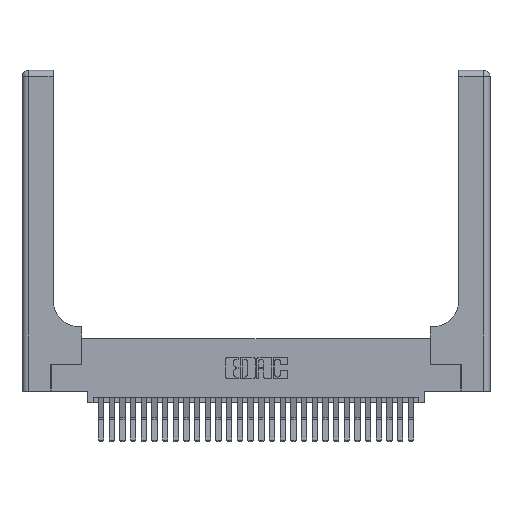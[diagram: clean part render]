
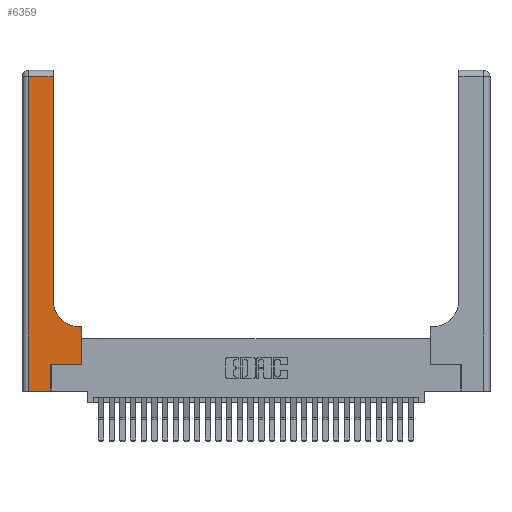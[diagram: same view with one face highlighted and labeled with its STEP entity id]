
A CAD part, top view. The second image highlights one B-rep face of the part: STEP entity #6359.
In plain terms, the highlighted planar face has unit normal (0, 0, 1).
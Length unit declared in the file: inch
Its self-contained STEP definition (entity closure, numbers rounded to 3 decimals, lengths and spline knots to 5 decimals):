
#84 = LINE ( 'NONE', #16524, #6353 ) ;
#564 = PLANE ( 'NONE',  #16732 ) ;
#703 = DIRECTION ( 'NONE',  ( 0., 1., 0. ) ) ;
#1130 = FACE_OUTER_BOUND ( 'NONE', #27902, .T. ) ;
#1442 = EDGE_CURVE ( 'NONE', #24325, #23639, #12715, .T. ) ;
#1774 = VERTEX_POINT ( 'NONE', #27814 ) ;
#1935 = DIRECTION ( 'NONE',  ( 1., 0., 0. ) ) ;
#2265 = DIRECTION ( 'NONE',  ( 1., 0., 0. ) ) ;
#2338 = CARTESIAN_POINT ( 'NONE',  ( 0., 2.94, 0.37 ) ) ;
#2570 = DIRECTION ( 'NONE',  ( -1., 0., 0. ) ) ;
#2942 = DIRECTION ( 'NONE',  ( 1., 0., 0. ) ) ;
#3468 = EDGE_CURVE ( 'NONE', #24528, #9712, #16293, .T. ) ;
#4187 = DIRECTION ( 'NONE',  ( 0., 0., -1. ) ) ;
#5060 = LINE ( 'NONE', #18318, #6574 ) ;
#5569 = EDGE_CURVE ( 'NONE', #18376, #21443, #25227, .T. ) ;
#5660 = ORIENTED_EDGE ( 'NONE', *, *, #5751, .T. ) ;
#5750 = CARTESIAN_POINT ( 'NONE',  ( 0.06, 2.94, 0.37 ) ) ;
#5751 = EDGE_CURVE ( 'NONE', #23639, #13401, #20760, .T. ) ;
#6353 = VECTOR ( 'NONE', #11831, 39.37008 ) ;
#6359 = ADVANCED_FACE ( 'NONE', ( #1130 ), #564, .F. ) ;
#6574 = VECTOR ( 'NONE', #25292, 39.37008 ) ;
#6883 = ORIENTED_EDGE ( 'NONE', *, *, #17012, .T. ) ;
#7183 = DIRECTION ( 'NONE',  ( -1., 0., 0. ) ) ;
#8137 = VECTOR ( 'NONE', #23333, 39.37008 ) ;
#9130 = ORIENTED_EDGE ( 'NONE', *, *, #1442, .T. ) ;
#9712 = VERTEX_POINT ( 'NONE', #17185 ) ;
#9992 = ORIENTED_EDGE ( 'NONE', *, *, #3468, .T. ) ;
#10165 = CARTESIAN_POINT ( 'NONE',  ( 0.269, 0., 0.37 ) ) ;
#10374 = VECTOR ( 'NONE', #2942, 39.37008 ) ;
#11231 = VECTOR ( 'NONE', #7183, 39.37008 ) ;
#11486 = EDGE_CURVE ( 'NONE', #21443, #1774, #5060, .T. ) ;
#11831 = DIRECTION ( 'NONE',  ( 0., 1., 0. ) ) ;
#11930 = CARTESIAN_POINT ( 'NONE',  ( 0.269, 0., 0.37 ) ) ;
#12715 = LINE ( 'NONE', #2338, #11231 ) ;
#13367 = CARTESIAN_POINT ( 'NONE',  ( 0.269, 0.25, 0.37 ) ) ;
#13401 = VERTEX_POINT ( 'NONE', #15048 ) ;
#13460 = CARTESIAN_POINT ( 'NONE',  ( 0., 3., 0.37 ) ) ;
#13659 = EDGE_CURVE ( 'NONE', #13401, #16905, #27153, .T. ) ;
#13711 = AXIS2_PLACEMENT_3D ( 'NONE', #16395, #21359, #2265 ) ;
#13730 = ORIENTED_EDGE ( 'NONE', *, *, #25328, .T. ) ;
#13891 = CARTESIAN_POINT ( 'NONE',  ( 0.06, 3., 0.37 ) ) ;
#14694 = CARTESIAN_POINT ( 'NONE',  ( 0.269, 0.25, 0.37 ) ) ;
#14718 = ORIENTED_EDGE ( 'NONE', *, *, #13659, .T. ) ;
#15048 = CARTESIAN_POINT ( 'NONE',  ( 0.06, 0., 0.37 ) ) ;
#15854 = CARTESIAN_POINT ( 'NONE',  ( 0.5415, 0.6, 0.37 ) ) ;
#15984 = CARTESIAN_POINT ( 'NONE',  ( 0., 0., 0.37 ) ) ;
#16197 = LINE ( 'NONE', #25303, #27287 ) ;
#16293 = CIRCLE ( 'NONE', #13711, 0.25 ) ;
#16395 = CARTESIAN_POINT ( 'NONE',  ( 0.5415, 0.85, 0.37 ) ) ;
#16524 = CARTESIAN_POINT ( 'NONE',  ( 0.2915, 3., 0.37 ) ) ;
#16732 = AXIS2_PLACEMENT_3D ( 'NONE', #13460, #4187, #2570 ) ;
#16905 = VERTEX_POINT ( 'NONE', #11930 ) ;
#17012 = EDGE_CURVE ( 'NONE', #16905, #18376, #19892, .T. ) ;
#17185 = CARTESIAN_POINT ( 'NONE',  ( 0.2915, 0.85, 0.37 ) ) ;
#17292 = EDGE_CURVE ( 'NONE', #1774, #24528, #16197, .T. ) ;
#18318 = CARTESIAN_POINT ( 'NONE',  ( 0.5585, 0.25, 0.37 ) ) ;
#18376 = VERTEX_POINT ( 'NONE', #13367 ) ;
#18753 = ORIENTED_EDGE ( 'NONE', *, *, #5569, .T. ) ;
#19892 = LINE ( 'NONE', #10165, #25860 ) ;
#20760 = LINE ( 'NONE', #13891, #8137 ) ;
#21112 = CARTESIAN_POINT ( 'NONE',  ( 0.5585, 0.25, 0.37 ) ) ;
#21359 = DIRECTION ( 'NONE',  ( 0., 0., -1. ) ) ;
#21443 = VERTEX_POINT ( 'NONE', #21112 ) ;
#23333 = DIRECTION ( 'NONE',  ( 0., -1., 0. ) ) ;
#23639 = VERTEX_POINT ( 'NONE', #5750 ) ;
#24325 = VERTEX_POINT ( 'NONE', #29171 ) ;
#24528 = VERTEX_POINT ( 'NONE', #15854 ) ;
#25227 = LINE ( 'NONE', #14694, #10374 ) ;
#25292 = DIRECTION ( 'NONE',  ( 0., 1., 0. ) ) ;
#25303 = CARTESIAN_POINT ( 'NONE',  ( 0.2915, 0.6, 0.37 ) ) ;
#25328 = EDGE_CURVE ( 'NONE', #9712, #24325, #84, .T. ) ;
#25860 = VECTOR ( 'NONE', #703, 39.37008 ) ;
#26413 = VECTOR ( 'NONE', #1935, 39.37008 ) ;
#27153 = LINE ( 'NONE', #15984, #26413 ) ;
#27287 = VECTOR ( 'NONE', #27667, 39.37008 ) ;
#27667 = DIRECTION ( 'NONE',  ( -1., 0., 0. ) ) ;
#27814 = CARTESIAN_POINT ( 'NONE',  ( 0.5585, 0.6, 0.37 ) ) ;
#27902 = EDGE_LOOP ( 'NONE', ( #13730, #9130, #5660, #14718, #6883, #18753, #29709, #29201, #9992 ) ) ;
#29171 = CARTESIAN_POINT ( 'NONE',  ( 0.2915, 2.94, 0.37 ) ) ;
#29201 = ORIENTED_EDGE ( 'NONE', *, *, #17292, .T. ) ;
#29709 = ORIENTED_EDGE ( 'NONE', *, *, #11486, .T. ) ;
